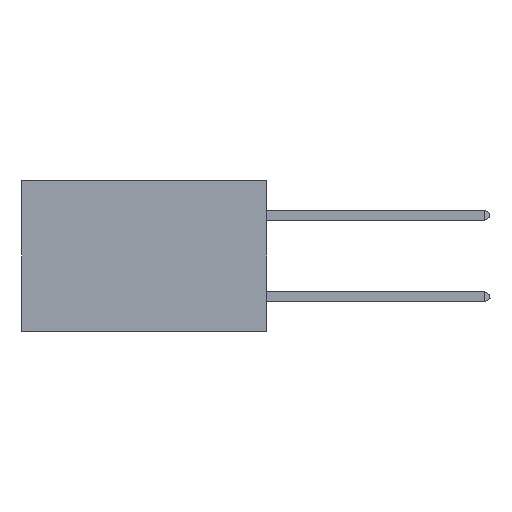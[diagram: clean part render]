
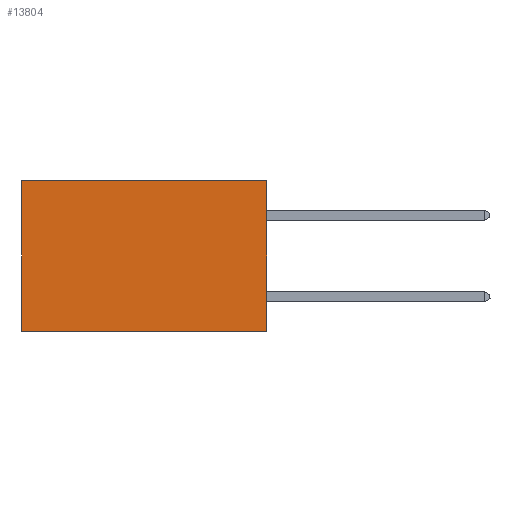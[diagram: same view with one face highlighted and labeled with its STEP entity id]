
A CAD part, left-side view. The second image highlights one B-rep face of the part: STEP entity #13804.
In plain terms, the highlighted planar face has unit normal (-1, 0, 0).
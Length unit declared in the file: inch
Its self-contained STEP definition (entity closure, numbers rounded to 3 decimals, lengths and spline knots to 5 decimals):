
#1174 = DIRECTION ( 'NONE',  ( 0., 1., 0. ) ) ;
#1757 = DIRECTION ( 'NONE',  ( 0., 1., 0. ) ) ;
#1934 = VERTEX_POINT ( 'NONE', #22366 ) ;
#3227 = CARTESIAN_POINT ( 'NONE',  ( 0.2875, 0., 0. ) ) ;
#3607 = LINE ( 'NONE', #22817, #21549 ) ;
#3660 = ORIENTED_EDGE ( 'NONE', *, *, #24691, .F. ) ;
#6528 = FACE_OUTER_BOUND ( 'NONE', #9040, .T. ) ;
#7265 = VERTEX_POINT ( 'NONE', #18006 ) ;
#8353 = CARTESIAN_POINT ( 'NONE',  ( 0.2875, 0., -0.37 ) ) ;
#8487 = AXIS2_PLACEMENT_3D ( 'NONE', #3227, #18851, #11024 ) ;
#8576 = ORIENTED_EDGE ( 'NONE', *, *, #20579, .T. ) ;
#9040 = EDGE_LOOP ( 'NONE', ( #9343, #10858, #3660, #8576 ) ) ;
#9046 = LINE ( 'NONE', #8353, #16141 ) ;
#9343 = ORIENTED_EDGE ( 'NONE', *, *, #23204, .T. ) ;
#9673 = CARTESIAN_POINT ( 'NONE',  ( 0.2875, 0., 0. ) ) ;
#9720 = LINE ( 'NONE', #9673, #23953 ) ;
#10753 = LINE ( 'NONE', #19713, #14792 ) ;
#10858 = ORIENTED_EDGE ( 'NONE', *, *, #13413, .F. ) ;
#11024 = DIRECTION ( 'NONE',  ( 0., 0., -1. ) ) ;
#11159 = DIRECTION ( 'NONE',  ( 0., 0., -1. ) ) ;
#11938 = CARTESIAN_POINT ( 'NONE',  ( 0.2875, 0.6, 0. ) ) ;
#11986 = DIRECTION ( 'NONE',  ( 0., 0., -1. ) ) ;
#12462 = VERTEX_POINT ( 'NONE', #14909 ) ;
#13413 = EDGE_CURVE ( 'NONE', #7265, #12462, #9046, .T. ) ;
#13804 = ADVANCED_FACE ( 'NONE', ( #6528 ), #17026, .F. ) ;
#14792 = VECTOR ( 'NONE', #11986, 39.37008 ) ;
#14909 = CARTESIAN_POINT ( 'NONE',  ( 0.2875, 0.6, -0.37 ) ) ;
#16141 = VECTOR ( 'NONE', #1174, 39.37008 ) ;
#17026 = PLANE ( 'NONE',  #8487 ) ;
#18006 = CARTESIAN_POINT ( 'NONE',  ( 0.2875, 0., -0.37 ) ) ;
#18851 = DIRECTION ( 'NONE',  ( 1., 0., 0. ) ) ;
#19713 = CARTESIAN_POINT ( 'NONE',  ( 0.2875, 0.6, 0. ) ) ;
#20579 = EDGE_CURVE ( 'NONE', #1934, #21374, #9720, .T. ) ;
#21374 = VERTEX_POINT ( 'NONE', #11938 ) ;
#21549 = VECTOR ( 'NONE', #11159, 39.37008 ) ;
#22366 = CARTESIAN_POINT ( 'NONE',  ( 0.2875, 0., 0. ) ) ;
#22817 = CARTESIAN_POINT ( 'NONE',  ( 0.2875, 0., 0. ) ) ;
#23204 = EDGE_CURVE ( 'NONE', #21374, #12462, #10753, .T. ) ;
#23953 = VECTOR ( 'NONE', #1757, 39.37008 ) ;
#24691 = EDGE_CURVE ( 'NONE', #1934, #7265, #3607, .T. ) ;
